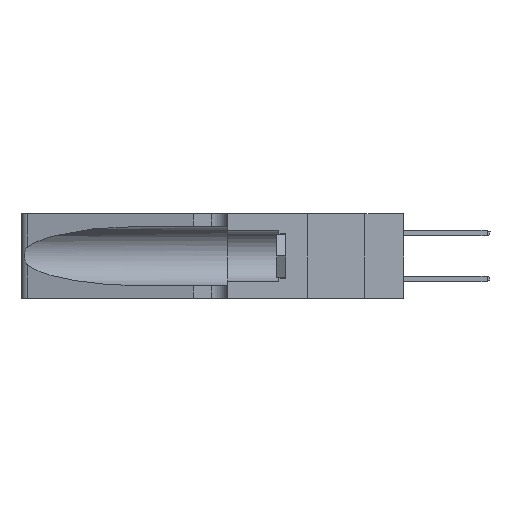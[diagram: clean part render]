
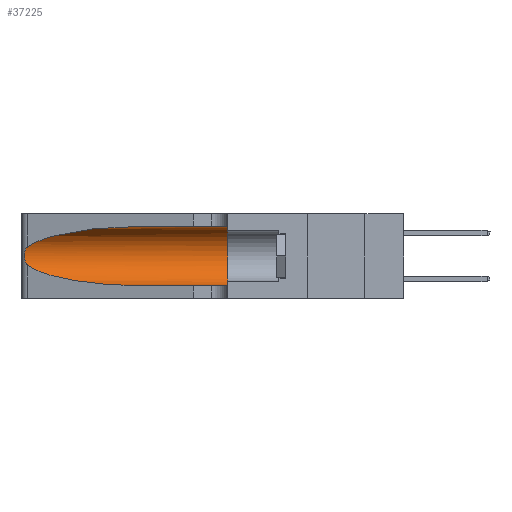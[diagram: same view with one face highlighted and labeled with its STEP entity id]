
A CAD part, left-side view. The second image highlights one B-rep face of the part: STEP entity #37225.
In plain terms, the highlighted cylindrical face has radius 3.308 mm (diameter 6.617 mm), a partial arc.
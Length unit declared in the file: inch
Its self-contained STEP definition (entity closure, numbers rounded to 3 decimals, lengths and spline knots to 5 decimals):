
#187 = ORIENTED_EDGE ( 'NONE', *, *, #39617, .T. ) ;
#194 = VECTOR ( 'NONE', #38589, 39.37008 ) ;
#2219 = DIRECTION ( 'NONE',  ( 0., 1., 0. ) ) ;
#2322 = FACE_OUTER_BOUND ( 'NONE', #29514, .T. ) ;
#3138 = ORIENTED_EDGE ( 'NONE', *, *, #35174, .T. ) ;
#3260 = CARTESIAN_POINT ( 'NONE',  ( 0.25639, 1.23184, 0.21858 ) ) ;
#3638 = DIRECTION ( 'NONE',  ( 0., -1., 0. ) ) ;
#4901 = AXIS2_PLACEMENT_3D ( 'NONE', #24060, #2219, #27697 ) ;
#5115 = CARTESIAN_POINT ( 'NONE',  ( 0.1305, 0.35, 0.05475 ) ) ;
#5323 = EDGE_CURVE ( 'NONE', #27414, #7996, #9849, .T. ) ;
#5894 = AXIS2_PLACEMENT_3D ( 'NONE', #35227, #27951, #31580 ) ;
#6974 = CARTESIAN_POINT ( 'NONE',  ( 0.25854, 1.2359, 0.20912 ) ) ;
#7996 = VERTEX_POINT ( 'NONE', #5115 ) ;
#9569 = CARTESIAN_POINT ( 'NONE',  ( 0.18966, 0.96281, 0.05475 ) ) ;
#9849 = CIRCLE ( 'NONE', #4901, 0.13025 ) ;
#10005 = LINE ( 'NONE', #16931, #194 ) ;
#10643 = CARTESIAN_POINT ( 'NONE',  ( 0.26075, 1.23896, 0.19203 ) ) ;
#13088 = CARTESIAN_POINT ( 'NONE',  ( 0.25487, 1.22718, 0.14631 ) ) ;
#14310 = CARTESIAN_POINT ( 'NONE',  ( 0.26017, 1.23833, 0.17102 ) ) ;
#16878 = ORIENTED_EDGE ( 'NONE', *, *, #5323, .F. ) ;
#16931 = CARTESIAN_POINT ( 'NONE',  ( 0.1305, 1.61858, 0.31525 ) ) ;
#17539 = CARTESIAN_POINT ( 'NONE',  ( 0.18966, 0.96281, 0.31525 ) ) ;
#17966 = CARTESIAN_POINT ( 'NONE',  ( 0.25789, 1.23486, 0.15765 ) ) ;
#19034 = VERTEX_POINT ( 'NONE', #39143 ) ;
#20631 = CYLINDRICAL_SURFACE ( 'NONE', #5894, 0.13025 ) ;
#21187 = CARTESIAN_POINT ( 'NONE',  ( 0.1305, 0.72297, 0.31525 ) ) ;
#21626 = CARTESIAN_POINT ( 'NONE',  ( 0.25555, 1.22993, 0.14849 ) ) ;
#24060 = CARTESIAN_POINT ( 'NONE',  ( 0.1305, 0.35, 0.185 ) ) ;
#24581 = EDGE_CURVE ( 'NONE', #25208, #38952, #30039, .T. ) ;
#24806 = CARTESIAN_POINT ( 'NONE',  ( 0.25487, 1.22718, 0.22369 ) ) ;
#25208 = VERTEX_POINT ( 'NONE', #38964 ) ;
#25474 = CARTESIAN_POINT ( 'NONE',  ( 0.1305, 1.61858, 0.05475 ) ) ;
#26578 = B_SPLINE_CURVE_WITH_KNOTS ( 'NONE', 3,
 ( #46630, #43077, #3260, #28705, #6974, #32356, #10643, #35986, #14310, #39625, #17966, #43234, #21626, #46801 ),
 .UNSPECIFIED., .F., .F.,
 ( 4, 2, 2, 2, 2, 2, 4 ),
 ( 0., 0.00027, 0.00053, 0.00107, 0.0016, 0.00187, 0.00214 ),
 .UNSPECIFIED. ) ;
#26738 = VECTOR ( 'NONE', #3638, 39.37008 ) ;
#27414 = VERTEX_POINT ( 'NONE', #45512 ) ;
#27648 = CARTESIAN_POINT ( 'NONE',  ( 0.2373, 1.15595, 0.08982 ) ) ;
#27697 = DIRECTION ( 'NONE',  ( 0., 0., 1. ) ) ;
#27872 = LINE ( 'NONE', #25474, #26738 ) ;
#27951 = DIRECTION ( 'NONE',  ( 0., -1., 0. ) ) ;
#28705 = CARTESIAN_POINT ( 'NONE',  ( 0.25787, 1.23484, 0.2124 ) ) ;
#29514 = EDGE_LOOP ( 'NONE', ( #34833, #187, #3138, #32021, #16878, #40104 ) ) ;
#30039 =( BOUNDED_CURVE ( )  B_SPLINE_CURVE ( 3, ( #21187, #17539, #46374, #24806 ),
 .UNSPECIFIED., .F., .F. ) 
 B_SPLINE_CURVE_WITH_KNOTS ( ( 4, 4 ),
 ( 1.5708, 2.84003 ),
 .UNSPECIFIED. ) 
 CURVE ( )  GEOMETRIC_REPRESENTATION_ITEM ( )  RATIONAL_B_SPLINE_CURVE ( ( 1., 0.87, 0.87, 1. ) ) 
 REPRESENTATION_ITEM ( '' )  );
#31580 = DIRECTION ( 'NONE',  ( 0., 0., -1. ) ) ;
#32021 = ORIENTED_EDGE ( 'NONE', *, *, #40910, .T. ) ;
#32356 = CARTESIAN_POINT ( 'NONE',  ( 0.26018, 1.23835, 0.19895 ) ) ;
#34833 = ORIENTED_EDGE ( 'NONE', *, *, #24581, .T. ) ;
#34917 = CARTESIAN_POINT ( 'NONE',  ( 0.1305, 0.72297, 0.05475 ) ) ;
#34980 =( BOUNDED_CURVE ( )  B_SPLINE_CURVE ( 3, ( #45591, #27648, #9569, #34917 ),
 .UNSPECIFIED., .F., .F. ) 
 B_SPLINE_CURVE_WITH_KNOTS ( ( 4, 4 ),
 ( 3.44316, 4.71239 ),
 .UNSPECIFIED. ) 
 CURVE ( )  GEOMETRIC_REPRESENTATION_ITEM ( )  RATIONAL_B_SPLINE_CURVE ( ( 1., 0.87, 0.87, 1. ) ) 
 REPRESENTATION_ITEM ( '' )  );
#35174 = EDGE_CURVE ( 'NONE', #40621, #19034, #34980, .T. ) ;
#35227 = CARTESIAN_POINT ( 'NONE',  ( 0.1305, 1.61858, 0.185 ) ) ;
#35986 = CARTESIAN_POINT ( 'NONE',  ( 0.26075, 1.23896, 0.178 ) ) ;
#36969 = CARTESIAN_POINT ( 'NONE',  ( 0.25487, 1.22718, 0.22369 ) ) ;
#37225 = ADVANCED_FACE ( 'NONE', ( #2322 ), #20631, .F. ) ;
#38589 = DIRECTION ( 'NONE',  ( 0., -1., 0. ) ) ;
#38952 = VERTEX_POINT ( 'NONE', #36969 ) ;
#38964 = CARTESIAN_POINT ( 'NONE',  ( 0.1305, 0.72297, 0.31525 ) ) ;
#39143 = CARTESIAN_POINT ( 'NONE',  ( 0.1305, 0.72297, 0.05475 ) ) ;
#39617 = EDGE_CURVE ( 'NONE', #38952, #40621, #26578, .T. ) ;
#39625 = CARTESIAN_POINT ( 'NONE',  ( 0.25856, 1.23593, 0.16098 ) ) ;
#40104 = ORIENTED_EDGE ( 'NONE', *, *, #45732, .F. ) ;
#40621 = VERTEX_POINT ( 'NONE', #13088 ) ;
#40910 = EDGE_CURVE ( 'NONE', #19034, #7996, #27872, .T. ) ;
#43077 = CARTESIAN_POINT ( 'NONE',  ( 0.25555, 1.22994, 0.2215 ) ) ;
#43234 = CARTESIAN_POINT ( 'NONE',  ( 0.25639, 1.23186, 0.15144 ) ) ;
#45512 = CARTESIAN_POINT ( 'NONE',  ( 0.1305, 0.35, 0.31525 ) ) ;
#45591 = CARTESIAN_POINT ( 'NONE',  ( 0.25487, 1.22718, 0.14631 ) ) ;
#45732 = EDGE_CURVE ( 'NONE', #25208, #27414, #10005, .T. ) ;
#46374 = CARTESIAN_POINT ( 'NONE',  ( 0.2373, 1.15595, 0.28018 ) ) ;
#46630 = CARTESIAN_POINT ( 'NONE',  ( 0.25487, 1.22718, 0.22369 ) ) ;
#46801 = CARTESIAN_POINT ( 'NONE',  ( 0.25487, 1.22718, 0.14631 ) ) ;
